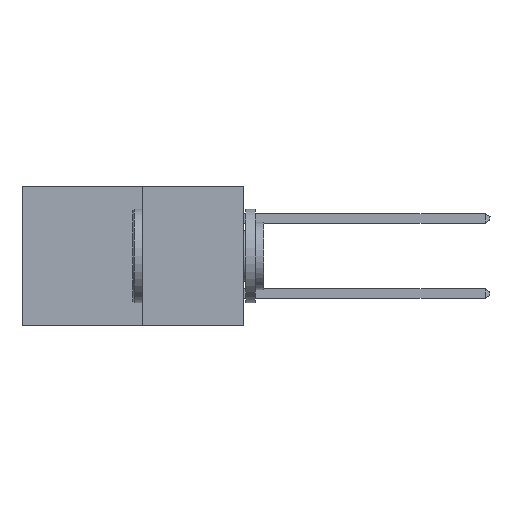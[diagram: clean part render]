
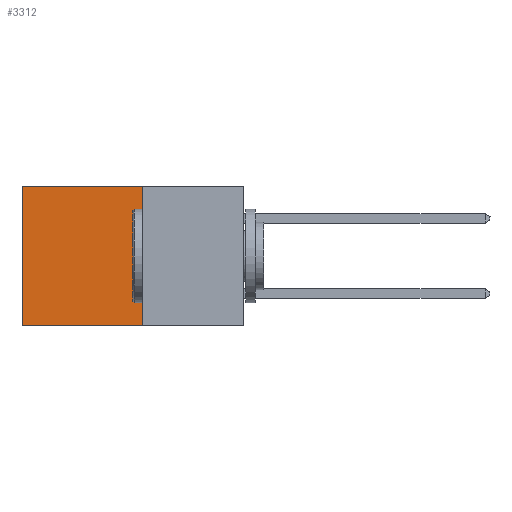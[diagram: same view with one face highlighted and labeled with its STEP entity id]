
A CAD part, left-side view. The second image highlights one B-rep face of the part: STEP entity #3312.
In plain terms, the highlighted planar face has unit normal (-1, 0, 0).
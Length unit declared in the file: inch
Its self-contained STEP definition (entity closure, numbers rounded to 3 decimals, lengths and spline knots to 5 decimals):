
#419 = CARTESIAN_POINT ( 'NONE',  ( 0.277, 0.59, -0.37 ) ) ;
#429 = CARTESIAN_POINT ( 'NONE',  ( 0.277, 0.59, -0.37 ) ) ;
#469 = EDGE_CURVE ( 'NONE', #3030, #2875, #6439, .T. ) ;
#598 = ORIENTED_EDGE ( 'NONE', *, *, #469, .F. ) ;
#987 = DIRECTION ( 'NONE',  ( 0., 0., -1. ) ) ;
#1164 = DIRECTION ( 'NONE',  ( 0., 0., -1. ) ) ;
#1190 = DIRECTION ( 'NONE',  ( 1., 0., 0. ) ) ;
#1372 = PLANE ( 'NONE',  #5130 ) ;
#1413 = CARTESIAN_POINT ( 'NONE',  ( 0.277, 0.27, -0.37 ) ) ;
#2318 = DIRECTION ( 'NONE',  ( 0., 1., 0. ) ) ;
#2397 = VECTOR ( 'NONE', #2318, 39.37008 ) ;
#2523 = EDGE_CURVE ( 'NONE', #7957, #3030, #5087, .T. ) ;
#2875 = VERTEX_POINT ( 'NONE', #419 ) ;
#3030 = VERTEX_POINT ( 'NONE', #4219 ) ;
#3048 = VECTOR ( 'NONE', #987, 39.37008 ) ;
#3312 = ADVANCED_FACE ( 'NONE', ( #6580 ), #1372, .F. ) ;
#3964 = LINE ( 'NONE', #429, #7486 ) ;
#4219 = CARTESIAN_POINT ( 'NONE',  ( 0.277, 0.27, -0.37 ) ) ;
#4438 = VECTOR ( 'NONE', #8503, 39.37008 ) ;
#5087 = LINE ( 'NONE', #7326, #3048 ) ;
#5130 = AXIS2_PLACEMENT_3D ( 'NONE', #1413, #1190, #1164 ) ;
#5257 = VERTEX_POINT ( 'NONE', #8090 ) ;
#5614 = CARTESIAN_POINT ( 'NONE',  ( 0.277, 0.27, -0.37 ) ) ;
#6047 = EDGE_LOOP ( 'NONE', ( #6579, #598, #8043, #8956 ) ) ;
#6329 = LINE ( 'NONE', #7146, #4438 ) ;
#6423 = EDGE_CURVE ( 'NONE', #5257, #2875, #3964, .T. ) ;
#6439 = LINE ( 'NONE', #5614, #2397 ) ;
#6579 = ORIENTED_EDGE ( 'NONE', *, *, #6423, .T. ) ;
#6580 = FACE_OUTER_BOUND ( 'NONE', #6047, .T. ) ;
#7146 = CARTESIAN_POINT ( 'NONE',  ( 0.277, 0.27, 0. ) ) ;
#7326 = CARTESIAN_POINT ( 'NONE',  ( 0.277, 0.27, -0.37 ) ) ;
#7450 = EDGE_CURVE ( 'NONE', #7957, #5257, #6329, .T. ) ;
#7486 = VECTOR ( 'NONE', #7859, 39.37008 ) ;
#7859 = DIRECTION ( 'NONE',  ( 0., 0., -1. ) ) ;
#7957 = VERTEX_POINT ( 'NONE', #8818 ) ;
#8043 = ORIENTED_EDGE ( 'NONE', *, *, #2523, .F. ) ;
#8090 = CARTESIAN_POINT ( 'NONE',  ( 0.277, 0.59, 0. ) ) ;
#8503 = DIRECTION ( 'NONE',  ( 0., 1., 0. ) ) ;
#8818 = CARTESIAN_POINT ( 'NONE',  ( 0.277, 0.27, 0. ) ) ;
#8956 = ORIENTED_EDGE ( 'NONE', *, *, #7450, .T. ) ;
